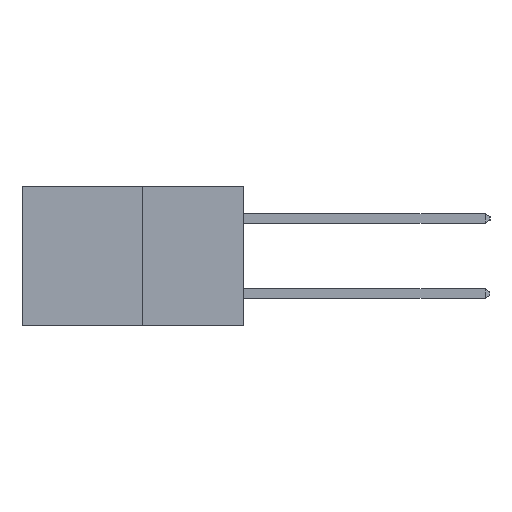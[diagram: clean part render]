
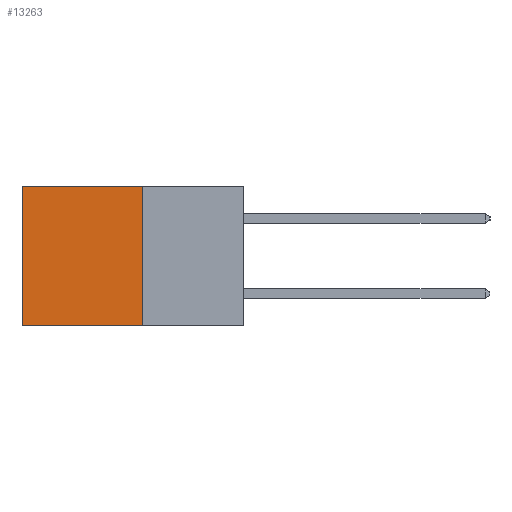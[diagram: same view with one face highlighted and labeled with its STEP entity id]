
A CAD part, left-side view. The second image highlights one B-rep face of the part: STEP entity #13263.
In plain terms, the highlighted planar face has unit normal (-1, 0, 0).
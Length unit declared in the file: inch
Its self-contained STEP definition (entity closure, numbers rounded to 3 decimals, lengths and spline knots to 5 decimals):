
#116 = VECTOR ( 'NONE', #12678, 39.37008 ) ;
#367 = DIRECTION ( 'NONE',  ( 0., 0., -1. ) ) ;
#616 = VECTOR ( 'NONE', #15924, 39.37008 ) ;
#679 = LINE ( 'NONE', #7517, #116 ) ;
#2046 = CARTESIAN_POINT ( 'NONE',  ( 0.277, 0.27, 0. ) ) ;
#2095 = CARTESIAN_POINT ( 'NONE',  ( 0.277, 0.27, -0.37 ) ) ;
#2694 = VERTEX_POINT ( 'NONE', #5690 ) ;
#5690 = CARTESIAN_POINT ( 'NONE',  ( 0.277, 0.59, 0. ) ) ;
#6436 = ORIENTED_EDGE ( 'NONE', *, *, #12487, .T. ) ;
#6629 = LINE ( 'NONE', #2095, #10697 ) ;
#7192 = VECTOR ( 'NONE', #9554, 39.37008 ) ;
#7481 = CARTESIAN_POINT ( 'NONE',  ( 0.277, 0.59, -0.37 ) ) ;
#7517 = CARTESIAN_POINT ( 'NONE',  ( 0.277, 0.59, -0.37 ) ) ;
#7810 = CARTESIAN_POINT ( 'NONE',  ( 0.277, 0.27, 0. ) ) ;
#8544 = VERTEX_POINT ( 'NONE', #2046 ) ;
#9198 = EDGE_CURVE ( 'NONE', #2694, #13069, #679, .T. ) ;
#9554 = DIRECTION ( 'NONE',  ( 0., 1., 0. ) ) ;
#9697 = CARTESIAN_POINT ( 'NONE',  ( 0.277, 0.27, -0.37 ) ) ;
#10346 = VERTEX_POINT ( 'NONE', #20433 ) ;
#10537 = LINE ( 'NONE', #17571, #616 ) ;
#10560 = EDGE_CURVE ( 'NONE', #10346, #13069, #10537, .T. ) ;
#10697 = VECTOR ( 'NONE', #367, 39.37008 ) ;
#11379 = DIRECTION ( 'NONE',  ( 0., 0., -1. ) ) ;
#12487 = EDGE_CURVE ( 'NONE', #8544, #2694, #20772, .T. ) ;
#12678 = DIRECTION ( 'NONE',  ( 0., 0., -1. ) ) ;
#13069 = VERTEX_POINT ( 'NONE', #7481 ) ;
#13263 = ADVANCED_FACE ( 'NONE', ( #18352 ), #19779, .F. ) ;
#15045 = ORIENTED_EDGE ( 'NONE', *, *, #9198, .T. ) ;
#15054 = EDGE_LOOP ( 'NONE', ( #15045, #21598, #18953, #6436 ) ) ;
#15924 = DIRECTION ( 'NONE',  ( 0., 1., 0. ) ) ;
#17306 = EDGE_CURVE ( 'NONE', #8544, #10346, #6629, .T. ) ;
#17569 = AXIS2_PLACEMENT_3D ( 'NONE', #9697, #21512, #11379 ) ;
#17571 = CARTESIAN_POINT ( 'NONE',  ( 0.277, 0.27, -0.37 ) ) ;
#18352 = FACE_OUTER_BOUND ( 'NONE', #15054, .T. ) ;
#18953 = ORIENTED_EDGE ( 'NONE', *, *, #17306, .F. ) ;
#19779 = PLANE ( 'NONE',  #17569 ) ;
#20433 = CARTESIAN_POINT ( 'NONE',  ( 0.277, 0.27, -0.37 ) ) ;
#20772 = LINE ( 'NONE', #7810, #7192 ) ;
#21512 = DIRECTION ( 'NONE',  ( 1., 0., 0. ) ) ;
#21598 = ORIENTED_EDGE ( 'NONE', *, *, #10560, .F. ) ;
